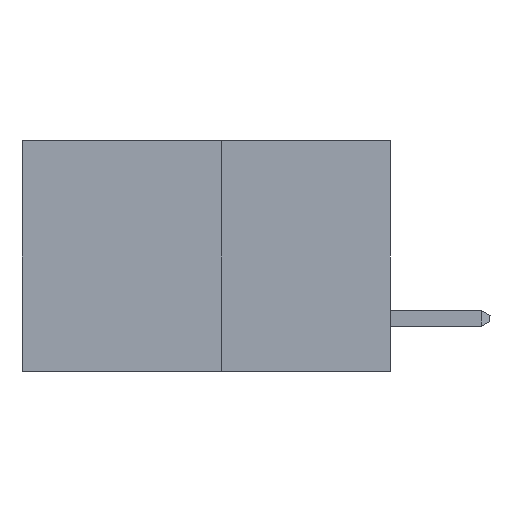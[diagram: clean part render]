
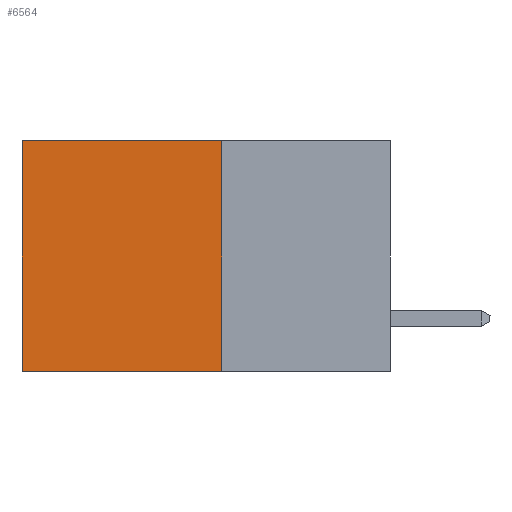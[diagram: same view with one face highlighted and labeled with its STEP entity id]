
A CAD part, left-side view. The second image highlights one B-rep face of the part: STEP entity #6564.
In plain terms, the highlighted planar face has unit normal (-1, 0, 0).
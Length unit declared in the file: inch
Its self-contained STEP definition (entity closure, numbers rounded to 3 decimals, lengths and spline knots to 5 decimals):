
#460 = CARTESIAN_POINT ( 'NONE',  ( 0.277, 0.27, 0. ) ) ;
#750 = LINE ( 'NONE', #460, #6677 ) ;
#1520 = CARTESIAN_POINT ( 'NONE',  ( 0.277, 0.27, -0.37 ) ) ;
#1556 = DIRECTION ( 'NONE',  ( 0., 0., -1. ) ) ;
#1874 = LINE ( 'NONE', #7995, #13576 ) ;
#2240 = ORIENTED_EDGE ( 'NONE', *, *, #10056, .T. ) ;
#2282 = ORIENTED_EDGE ( 'NONE', *, *, #3297, .F. ) ;
#2466 = ORIENTED_EDGE ( 'NONE', *, *, #6146, .F. ) ;
#2498 = FACE_OUTER_BOUND ( 'NONE', #6435, .T. ) ;
#2508 = AXIS2_PLACEMENT_3D ( 'NONE', #7499, #6129, #6081 ) ;
#2532 = ORIENTED_EDGE ( 'NONE', *, *, #9602, .T. ) ;
#3297 = EDGE_CURVE ( 'NONE', #8543, #14625, #5421, .T. ) ;
#3603 = CARTESIAN_POINT ( 'NONE',  ( 0.277, 0.59, 0. ) ) ;
#4539 = DIRECTION ( 'NONE',  ( 0., 0., -1. ) ) ;
#5421 = LINE ( 'NONE', #7537, #14170 ) ;
#6081 = DIRECTION ( 'NONE',  ( 0., 0., -1. ) ) ;
#6129 = DIRECTION ( 'NONE',  ( 1., 0., 0. ) ) ;
#6146 = EDGE_CURVE ( 'NONE', #7286, #8543, #6231, .T. ) ;
#6230 = PLANE ( 'NONE',  #2508 ) ;
#6231 = LINE ( 'NONE', #1520, #14885 ) ;
#6435 = EDGE_LOOP ( 'NONE', ( #2240, #2282, #2466, #2532 ) ) ;
#6564 = ADVANCED_FACE ( 'NONE', ( #2498 ), #6230, .F. ) ;
#6574 = DIRECTION ( 'NONE',  ( 0., 1., 0. ) ) ;
#6677 = VECTOR ( 'NONE', #13357, 39.37008 ) ;
#7286 = VERTEX_POINT ( 'NONE', #10625 ) ;
#7499 = CARTESIAN_POINT ( 'NONE',  ( 0.277, 0.27, -0.37 ) ) ;
#7537 = CARTESIAN_POINT ( 'NONE',  ( 0.277, 0.27, -0.37 ) ) ;
#7995 = CARTESIAN_POINT ( 'NONE',  ( 0.277, 0.59, -0.37 ) ) ;
#8028 = VERTEX_POINT ( 'NONE', #3603 ) ;
#8543 = VERTEX_POINT ( 'NONE', #9084 ) ;
#8711 = CARTESIAN_POINT ( 'NONE',  ( 0.277, 0.59, -0.37 ) ) ;
#9084 = CARTESIAN_POINT ( 'NONE',  ( 0.277, 0.27, -0.37 ) ) ;
#9602 = EDGE_CURVE ( 'NONE', #7286, #8028, #750, .T. ) ;
#10056 = EDGE_CURVE ( 'NONE', #8028, #14625, #1874, .T. ) ;
#10625 = CARTESIAN_POINT ( 'NONE',  ( 0.277, 0.27, 0. ) ) ;
#13357 = DIRECTION ( 'NONE',  ( 0., 1., 0. ) ) ;
#13576 = VECTOR ( 'NONE', #4539, 39.37008 ) ;
#14170 = VECTOR ( 'NONE', #6574, 39.37008 ) ;
#14625 = VERTEX_POINT ( 'NONE', #8711 ) ;
#14885 = VECTOR ( 'NONE', #1556, 39.37008 ) ;
